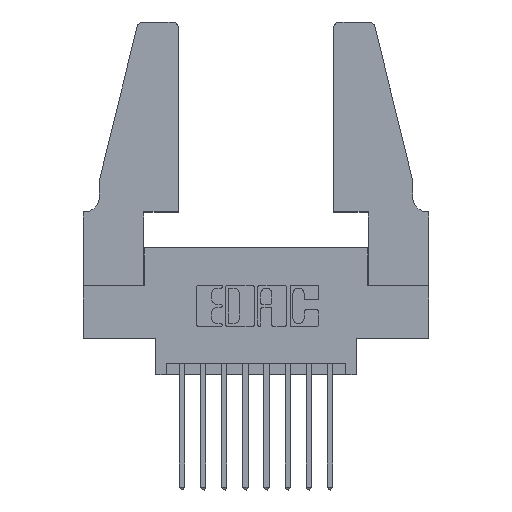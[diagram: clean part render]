
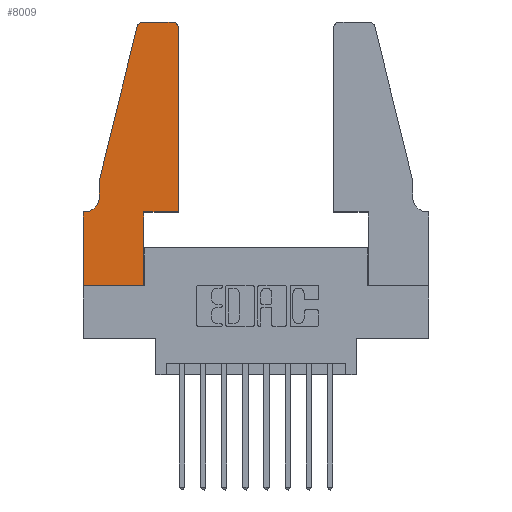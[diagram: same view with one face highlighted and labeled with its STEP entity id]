
A CAD part, top view. The second image highlights one B-rep face of the part: STEP entity #8009.
In plain terms, the highlighted planar face has unit normal (0, 0, 1).
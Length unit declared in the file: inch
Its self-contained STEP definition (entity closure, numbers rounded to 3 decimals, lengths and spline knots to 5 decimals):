
#76 = EDGE_CURVE ( 'NONE', #4985, #7144, #7633, .T. ) ;
#170 = LINE ( 'NONE', #11256, #5343 ) ;
#363 = FACE_OUTER_BOUND ( 'NONE', #2627, .T. ) ;
#388 = CARTESIAN_POINT ( 'NONE',  ( 0.284, 1.22, 0.37 ) ) ;
#678 = VECTOR ( 'NONE', #9311, 39.37008 ) ;
#683 = CARTESIAN_POINT ( 'NONE',  ( 0., 0., 0.37 ) ) ;
#823 = VECTOR ( 'NONE', #4772, 39.37008 ) ;
#894 = EDGE_CURVE ( 'NONE', #2992, #2950, #3764, .T. ) ;
#1441 = DIRECTION ( 'NONE',  ( 1., 0., 0. ) ) ;
#1682 = EDGE_CURVE ( 'NONE', #6849, #9997, #170, .T. ) ;
#1860 = ORIENTED_EDGE ( 'NONE', *, *, #1892, .T. ) ;
#1892 = EDGE_CURVE ( 'NONE', #4962, #4985, #3393, .T. ) ;
#1913 = EDGE_CURVE ( 'NONE', #7144, #6849, #11226, .T. ) ;
#2035 = ORIENTED_EDGE ( 'NONE', *, *, #1682, .T. ) ;
#2078 = DIRECTION ( 'NONE',  ( 1., 0., 0. ) ) ;
#2102 = CARTESIAN_POINT ( 'NONE',  ( 0.2865, 0., 0.37 ) ) ;
#2274 = DIRECTION ( 'NONE',  ( -1., 0., 0. ) ) ;
#2433 = EDGE_CURVE ( 'NONE', #7108, #3970, #9640, .T. ) ;
#2518 = EDGE_CURVE ( 'NONE', #5679, #4962, #6278, .T. ) ;
#2627 = EDGE_LOOP ( 'NONE', ( #7562, #5163, #10976, #1860, #4238, #12835, #2035, #8282, #11787, #5378, #9240, #5157 ) ) ;
#2674 = LINE ( 'NONE', #3200, #12820 ) ;
#2748 = CARTESIAN_POINT ( 'NONE',  ( 0.0055, 0.35, 0.37 ) ) ;
#2950 = VERTEX_POINT ( 'NONE', #11692 ) ;
#2992 = VERTEX_POINT ( 'NONE', #11355 ) ;
#3144 = DIRECTION ( 'NONE',  ( 0., 0., -1. ) ) ;
#3200 = CARTESIAN_POINT ( 'NONE',  ( 0.2865, 0.35, 0.37 ) ) ;
#3249 = CARTESIAN_POINT ( 'NONE',  ( 0.4505, 1.22, 0.37 ) ) ;
#3270 = EDGE_CURVE ( 'NONE', #9470, #7108, #9321, .T. ) ;
#3393 = LINE ( 'NONE', #4370, #678 ) ;
#3764 = LINE ( 'NONE', #8323, #6493 ) ;
#3970 = VERTEX_POINT ( 'NONE', #4937 ) ;
#4238 = ORIENTED_EDGE ( 'NONE', *, *, #76, .T. ) ;
#4325 = CARTESIAN_POINT ( 'NONE',  ( 0., 0.35, 0.37 ) ) ;
#4370 = CARTESIAN_POINT ( 'NONE',  ( 0.0755, 0.5, 0.37 ) ) ;
#4570 = CARTESIAN_POINT ( 'NONE',  ( 0.0055, 0.42, 0.37 ) ) ;
#4731 = CARTESIAN_POINT ( 'NONE',  ( 0.4205, 1.25, 0.37 ) ) ;
#4753 = CARTESIAN_POINT ( 'NONE',  ( 0.0755, 0.5, 0.37 ) ) ;
#4772 = DIRECTION ( 'NONE',  ( -0.239, -0.971, 0. ) ) ;
#4937 = CARTESIAN_POINT ( 'NONE',  ( 0.284, 1.25, 0.37 ) ) ;
#4962 = VERTEX_POINT ( 'NONE', #8240 ) ;
#4985 = VERTEX_POINT ( 'NONE', #7373 ) ;
#5157 = ORIENTED_EDGE ( 'NONE', *, *, #3270, .T. ) ;
#5163 = ORIENTED_EDGE ( 'NONE', *, *, #6981, .T. ) ;
#5260 = DIRECTION ( 'NONE',  ( 0., 1., 0. ) ) ;
#5343 = VECTOR ( 'NONE', #9106, 39.37008 ) ;
#5378 = ORIENTED_EDGE ( 'NONE', *, *, #894, .T. ) ;
#5679 = VERTEX_POINT ( 'NONE', #11632 ) ;
#5967 = DIRECTION ( 'NONE',  ( -1., 0., 0. ) ) ;
#5994 = CARTESIAN_POINT ( 'NONE',  ( 0.2605, 1.25, 0.37 ) ) ;
#6127 = PLANE ( 'NONE',  #10266 ) ;
#6278 = LINE ( 'NONE', #4753, #823 ) ;
#6393 = AXIS2_PLACEMENT_3D ( 'NONE', #9507, #9477, #9464 ) ;
#6493 = VECTOR ( 'NONE', #7655, 39.37008 ) ;
#6520 = VERTEX_POINT ( 'NONE', #2102 ) ;
#6652 = VECTOR ( 'NONE', #5260, 39.37008 ) ;
#6849 = VERTEX_POINT ( 'NONE', #4325 ) ;
#6850 = CIRCLE ( 'NONE', #6963, 0.03 ) ;
#6898 = AXIS2_PLACEMENT_3D ( 'NONE', #4570, #3144, #12217 ) ;
#6963 = AXIS2_PLACEMENT_3D ( 'NONE', #388, #7592, #1441 ) ;
#6981 = EDGE_CURVE ( 'NONE', #3970, #5679, #6850, .T. ) ;
#7108 = VERTEX_POINT ( 'NONE', #4731 ) ;
#7144 = VERTEX_POINT ( 'NONE', #2748 ) ;
#7168 = CARTESIAN_POINT ( 'NONE',  ( 0., 0.35, 0.37 ) ) ;
#7311 = DIRECTION ( 'NONE',  ( 0., 1., 0. ) ) ;
#7373 = CARTESIAN_POINT ( 'NONE',  ( 0.0755, 0.42, 0.37 ) ) ;
#7562 = ORIENTED_EDGE ( 'NONE', *, *, #2433, .T. ) ;
#7592 = DIRECTION ( 'NONE',  ( 0., 0., 1. ) ) ;
#7633 = CIRCLE ( 'NONE', #6898, 0.07 ) ;
#7655 = DIRECTION ( 'NONE',  ( 1., 0., 0. ) ) ;
#8003 = LINE ( 'NONE', #12595, #10354 ) ;
#8009 = ADVANCED_FACE ( 'NONE', ( #363 ), #6127, .T. ) ;
#8188 = DIRECTION ( 'NONE',  ( 0., 0., 1. ) ) ;
#8240 = CARTESIAN_POINT ( 'NONE',  ( 0.0755, 0.5, 0.37 ) ) ;
#8282 = ORIENTED_EDGE ( 'NONE', *, *, #9830, .T. ) ;
#8323 = CARTESIAN_POINT ( 'NONE',  ( 0.4505, 0.35, 0.37 ) ) ;
#8538 = VECTOR ( 'NONE', #2274, 39.37008 ) ;
#8646 = CARTESIAN_POINT ( 'NONE',  ( 0.0755, 0.35, 0.37 ) ) ;
#9050 = LINE ( 'NONE', #11342, #6652 ) ;
#9106 = DIRECTION ( 'NONE',  ( 0., -1., 0. ) ) ;
#9240 = ORIENTED_EDGE ( 'NONE', *, *, #12156, .T. ) ;
#9311 = DIRECTION ( 'NONE',  ( 0., -1., 0. ) ) ;
#9321 = CIRCLE ( 'NONE', #6393, 0.03 ) ;
#9464 = DIRECTION ( 'NONE',  ( 1., 0., 0. ) ) ;
#9470 = VERTEX_POINT ( 'NONE', #3249 ) ;
#9477 = DIRECTION ( 'NONE',  ( 0., 0., 1. ) ) ;
#9507 = CARTESIAN_POINT ( 'NONE',  ( 0.4205, 1.22, 0.37 ) ) ;
#9640 = LINE ( 'NONE', #5994, #12276 ) ;
#9830 = EDGE_CURVE ( 'NONE', #9997, #6520, #8003, .T. ) ;
#9997 = VERTEX_POINT ( 'NONE', #683 ) ;
#10266 = AXIS2_PLACEMENT_3D ( 'NONE', #7168, #8188, #2078 ) ;
#10354 = VECTOR ( 'NONE', #10653, 39.37008 ) ;
#10653 = DIRECTION ( 'NONE',  ( 1., 0., 0. ) ) ;
#10934 = EDGE_CURVE ( 'NONE', #6520, #2992, #2674, .T. ) ;
#10976 = ORIENTED_EDGE ( 'NONE', *, *, #2518, .T. ) ;
#11226 = LINE ( 'NONE', #8646, #8538 ) ;
#11256 = CARTESIAN_POINT ( 'NONE',  ( 0., 0., 0.37 ) ) ;
#11342 = CARTESIAN_POINT ( 'NONE',  ( 0.4505, 0.35, 0.37 ) ) ;
#11355 = CARTESIAN_POINT ( 'NONE',  ( 0.2865, 0.35, 0.37 ) ) ;
#11632 = CARTESIAN_POINT ( 'NONE',  ( 0.25487, 1.22718, 0.37 ) ) ;
#11692 = CARTESIAN_POINT ( 'NONE',  ( 0.4505, 0.35, 0.37 ) ) ;
#11787 = ORIENTED_EDGE ( 'NONE', *, *, #10934, .T. ) ;
#12156 = EDGE_CURVE ( 'NONE', #2950, #9470, #9050, .T. ) ;
#12217 = DIRECTION ( 'NONE',  ( -1., 0., 0. ) ) ;
#12276 = VECTOR ( 'NONE', #5967, 39.37008 ) ;
#12595 = CARTESIAN_POINT ( 'NONE',  ( 0., 0., 0.37 ) ) ;
#12820 = VECTOR ( 'NONE', #7311, 39.37008 ) ;
#12835 = ORIENTED_EDGE ( 'NONE', *, *, #1913, .T. ) ;
